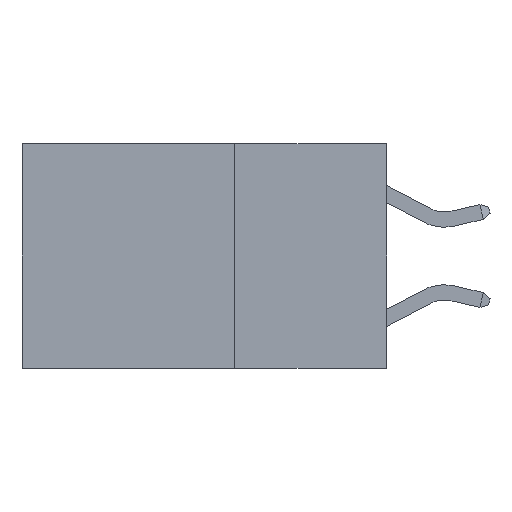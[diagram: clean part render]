
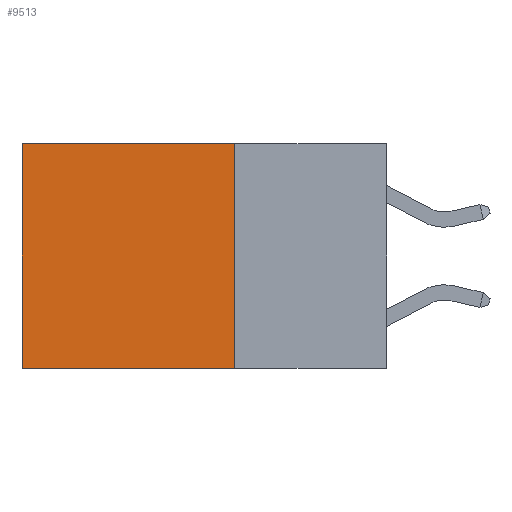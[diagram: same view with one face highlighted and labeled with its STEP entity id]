
A CAD part, left-side view. The second image highlights one B-rep face of the part: STEP entity #9513.
In plain terms, the highlighted planar face has unit normal (-1, 0, 0).
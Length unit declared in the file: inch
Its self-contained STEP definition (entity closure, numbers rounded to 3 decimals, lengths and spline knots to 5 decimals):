
#1830 = DIRECTION ( 'NONE',  ( 0., 1., 0. ) ) ;
#1887 = CARTESIAN_POINT ( 'NONE',  ( 0.2625, 0.25, 0. ) ) ;
#1953 = CARTESIAN_POINT ( 'NONE',  ( 0.2625, 0.25, 0. ) ) ;
#2081 = DIRECTION ( 'NONE',  ( 1., 0., 0. ) ) ;
#2104 = EDGE_LOOP ( 'NONE', ( #5826, #10481, #8882, #7399 ) ) ;
#2129 = DIRECTION ( 'NONE',  ( 0., 0., -1. ) ) ;
#2696 = VERTEX_POINT ( 'NONE', #7552 ) ;
#3177 = VECTOR ( 'NONE', #1830, 39.37008 ) ;
#3693 = CARTESIAN_POINT ( 'NONE',  ( 0.2625, 0.25, -0.37 ) ) ;
#3903 = DIRECTION ( 'NONE',  ( 0., 0., -1. ) ) ;
#4717 = DIRECTION ( 'NONE',  ( 0., 0., -1. ) ) ;
#5072 = CARTESIAN_POINT ( 'NONE',  ( 0.2625, 0.6, -0.37 ) ) ;
#5085 = EDGE_CURVE ( 'NONE', #10040, #11172, #10161, .T. ) ;
#5795 = EDGE_CURVE ( 'NONE', #10040, #2696, #9097, .T. ) ;
#5826 = ORIENTED_EDGE ( 'NONE', *, *, #9141, .T. ) ;
#6217 = VECTOR ( 'NONE', #2129, 39.37008 ) ;
#6616 = FACE_OUTER_BOUND ( 'NONE', #2104, .T. ) ;
#6670 = PLANE ( 'NONE',  #10208 ) ;
#7295 = VECTOR ( 'NONE', #3903, 39.37008 ) ;
#7307 = CARTESIAN_POINT ( 'NONE',  ( 0.2625, 0.25, 0. ) ) ;
#7399 = ORIENTED_EDGE ( 'NONE', *, *, #5795, .T. ) ;
#7552 = CARTESIAN_POINT ( 'NONE',  ( 0.2625, 0.6, 0. ) ) ;
#7592 = CARTESIAN_POINT ( 'NONE',  ( 0.2625, 0.6, 0. ) ) ;
#7595 = VERTEX_POINT ( 'NONE', #5072 ) ;
#7726 = EDGE_CURVE ( 'NONE', #11172, #7595, #9845, .T. ) ;
#8298 = CARTESIAN_POINT ( 'NONE',  ( 0.2625, 0.25, -0.37 ) ) ;
#8882 = ORIENTED_EDGE ( 'NONE', *, *, #5085, .F. ) ;
#9097 = LINE ( 'NONE', #7307, #11113 ) ;
#9141 = EDGE_CURVE ( 'NONE', #2696, #7595, #10292, .T. ) ;
#9513 = ADVANCED_FACE ( 'NONE', ( #6616 ), #6670, .F. ) ;
#9845 = LINE ( 'NONE', #8298, #3177 ) ;
#10040 = VERTEX_POINT ( 'NONE', #1887 ) ;
#10161 = LINE ( 'NONE', #11176, #7295 ) ;
#10208 = AXIS2_PLACEMENT_3D ( 'NONE', #1953, #2081, #4717 ) ;
#10235 = DIRECTION ( 'NONE',  ( 0., 1., 0. ) ) ;
#10292 = LINE ( 'NONE', #7592, #6217 ) ;
#10481 = ORIENTED_EDGE ( 'NONE', *, *, #7726, .F. ) ;
#11113 = VECTOR ( 'NONE', #10235, 39.37008 ) ;
#11172 = VERTEX_POINT ( 'NONE', #3693 ) ;
#11176 = CARTESIAN_POINT ( 'NONE',  ( 0.2625, 0.25, 0. ) ) ;
